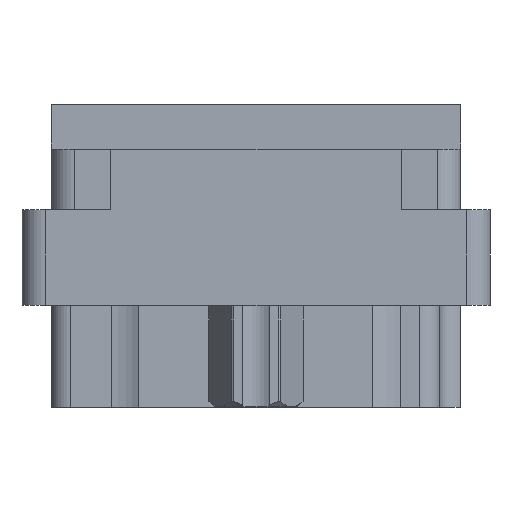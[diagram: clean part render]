
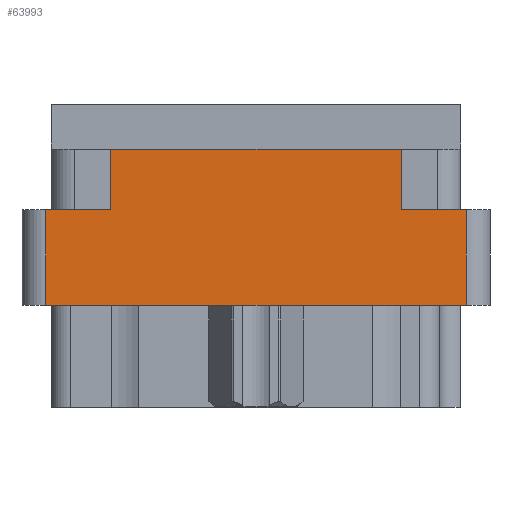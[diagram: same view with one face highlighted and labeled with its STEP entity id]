
A CAD part, left-side view. The second image highlights one B-rep face of the part: STEP entity #63993.
In plain terms, the highlighted planar face has unit normal (-1, 0, 0).
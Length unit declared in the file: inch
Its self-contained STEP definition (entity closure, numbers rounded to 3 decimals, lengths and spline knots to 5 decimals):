
#1705 = EDGE_CURVE ( 'NONE', #5358, #31329, #6188, .T. ) ;
#3952 = CARTESIAN_POINT ( 'NONE',  ( -1.359, 0., -0.277 ) ) ;
#3961 = DIRECTION ( 'NONE',  ( 0., 0., 1. ) ) ;
#5358 = VERTEX_POINT ( 'NONE', #20057 ) ;
#6188 = LINE ( 'NONE', #22830, #49492 ) ;
#8043 = PLANE ( 'NONE',  #56852 ) ;
#8255 = EDGE_CURVE ( 'NONE', #52504, #9760, #61810, .T. ) ;
#9408 = LINE ( 'NONE', #58457, #26462 ) ;
#9760 = VERTEX_POINT ( 'NONE', #59317 ) ;
#9907 = EDGE_CURVE ( 'NONE', #28997, #69631, #45833, .T. ) ;
#11861 = EDGE_CURVE ( 'NONE', #5358, #42353, #37136, .T. ) ;
#12189 = EDGE_CURVE ( 'NONE', #73696, #69631, #68118, .T. ) ;
#12531 = CARTESIAN_POINT ( 'NONE',  ( -1.359, 0.555, -0.529 ) ) ;
#15506 = DIRECTION ( 'NONE',  ( 0., 1., 0. ) ) ;
#15748 = CARTESIAN_POINT ( 'NONE',  ( -1.359, 0., -0.529 ) ) ;
#16516 = DIRECTION ( 'NONE',  ( 0., -1., 0. ) ) ;
#20057 = CARTESIAN_POINT ( 'NONE',  ( -1.359, 0.555, -0.277 ) ) ;
#21126 = VECTOR ( 'NONE', #49939, 39.37008 ) ;
#22830 = CARTESIAN_POINT ( 'NONE',  ( -1.359, 0., -0.277 ) ) ;
#24798 = CARTESIAN_POINT ( 'NONE',  ( -1.359, -0.3825, -0.277 ) ) ;
#25558 = CARTESIAN_POINT ( 'NONE',  ( -1.359, 0.3825, -0.277 ) ) ;
#25654 = CARTESIAN_POINT ( 'NONE',  ( -1.359, -0.555, -0.529 ) ) ;
#26246 = CARTESIAN_POINT ( 'NONE',  ( -1.359, -0.617, -0.798 ) ) ;
#26462 = VECTOR ( 'NONE', #3961, 39.37008 ) ;
#27732 = VECTOR ( 'NONE', #75972, 39.37008 ) ;
#28997 = VERTEX_POINT ( 'NONE', #37967 ) ;
#30676 = CARTESIAN_POINT ( 'NONE',  ( -1.359, 0.617, -0.117 ) ) ;
#31329 = VERTEX_POINT ( 'NONE', #25558 ) ;
#32830 = DIRECTION ( 'NONE',  ( 0., 0., 1. ) ) ;
#34398 = ORIENTED_EDGE ( 'NONE', *, *, #11861, .T. ) ;
#35774 = CARTESIAN_POINT ( 'NONE',  ( -1.359, -0.555, -0.798 ) ) ;
#37136 = LINE ( 'NONE', #43646, #21126 ) ;
#37967 = CARTESIAN_POINT ( 'NONE',  ( -1.359, 0.3825, -0.117 ) ) ;
#38644 = LINE ( 'NONE', #3952, #78217 ) ;
#39451 = ORIENTED_EDGE ( 'NONE', *, *, #68128, .F. ) ;
#40702 = CARTESIAN_POINT ( 'NONE',  ( -1.359, -0.3825, -0.277 ) ) ;
#42208 = DIRECTION ( 'NONE',  ( 0., -1., 0. ) ) ;
#42353 = VERTEX_POINT ( 'NONE', #12531 ) ;
#42512 = ORIENTED_EDGE ( 'NONE', *, *, #46922, .F. ) ;
#43646 = CARTESIAN_POINT ( 'NONE',  ( -1.359, 0.555, -0.798 ) ) ;
#45820 = VECTOR ( 'NONE', #15506, 39.37008 ) ;
#45833 = LINE ( 'NONE', #30676, #48712 ) ;
#46922 = EDGE_CURVE ( 'NONE', #31329, #28997, #9408, .T. ) ;
#48712 = VECTOR ( 'NONE', #42208, 39.37008 ) ;
#49492 = VECTOR ( 'NONE', #16516, 39.37008 ) ;
#49939 = DIRECTION ( 'NONE',  ( 0., 0., -1. ) ) ;
#51672 = ORIENTED_EDGE ( 'NONE', *, *, #12189, .T. ) ;
#52351 = EDGE_LOOP ( 'NONE', ( #54814, #34398, #57403, #77610, #39451, #51672, #54831, #42512 ) ) ;
#52504 = VERTEX_POINT ( 'NONE', #25654 ) ;
#54814 = ORIENTED_EDGE ( 'NONE', *, *, #1705, .F. ) ;
#54831 = ORIENTED_EDGE ( 'NONE', *, *, #9907, .F. ) ;
#56852 = AXIS2_PLACEMENT_3D ( 'NONE', #26246, #62748, #32830 ) ;
#57115 = LINE ( 'NONE', #15748, #45820 ) ;
#57403 = ORIENTED_EDGE ( 'NONE', *, *, #73977, .F. ) ;
#58176 = DIRECTION ( 'NONE',  ( 0., -1., 0. ) ) ;
#58457 = CARTESIAN_POINT ( 'NONE',  ( -1.359, 0.3825, -0.277 ) ) ;
#59317 = CARTESIAN_POINT ( 'NONE',  ( -1.359, -0.555, -0.277 ) ) ;
#60931 = VECTOR ( 'NONE', #77873, 39.37008 ) ;
#61810 = LINE ( 'NONE', #35774, #60931 ) ;
#61865 = CARTESIAN_POINT ( 'NONE',  ( -1.359, -0.3825, -0.117 ) ) ;
#62748 = DIRECTION ( 'NONE',  ( -1., 0., 0. ) ) ;
#63993 = ADVANCED_FACE ( 'NONE', ( #68399 ), #8043, .T. ) ;
#68118 = LINE ( 'NONE', #40702, #27732 ) ;
#68128 = EDGE_CURVE ( 'NONE', #73696, #9760, #38644, .T. ) ;
#68399 = FACE_OUTER_BOUND ( 'NONE', #52351, .T. ) ;
#69631 = VERTEX_POINT ( 'NONE', #61865 ) ;
#73696 = VERTEX_POINT ( 'NONE', #24798 ) ;
#73977 = EDGE_CURVE ( 'NONE', #52504, #42353, #57115, .T. ) ;
#75972 = DIRECTION ( 'NONE',  ( 0., 0., 1. ) ) ;
#77610 = ORIENTED_EDGE ( 'NONE', *, *, #8255, .T. ) ;
#77873 = DIRECTION ( 'NONE',  ( 0., 0., 1. ) ) ;
#78217 = VECTOR ( 'NONE', #58176, 39.37008 ) ;
